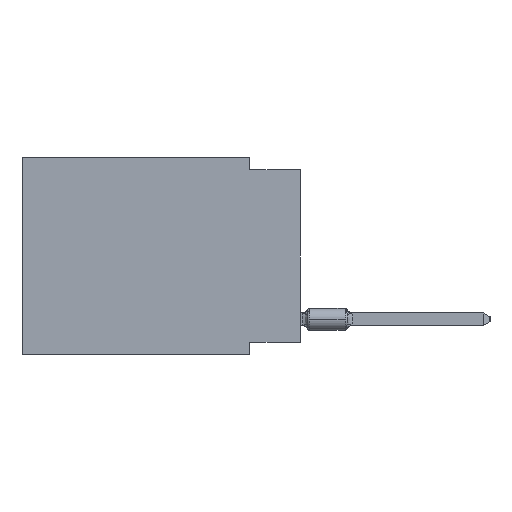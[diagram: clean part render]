
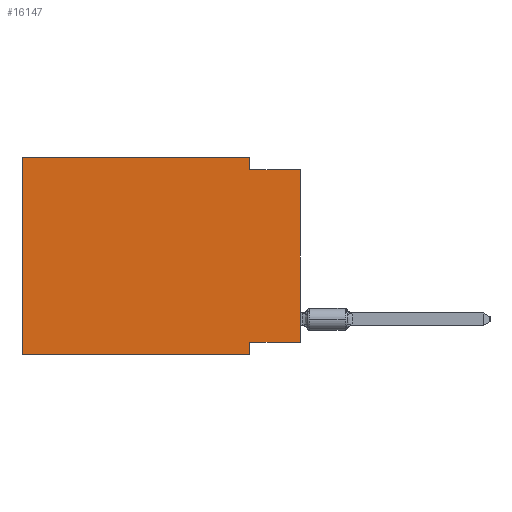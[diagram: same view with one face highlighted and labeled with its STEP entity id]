
A CAD part, left-side view. The second image highlights one B-rep face of the part: STEP entity #16147.
In plain terms, the highlighted planar face has unit normal (-1, 0, 0).
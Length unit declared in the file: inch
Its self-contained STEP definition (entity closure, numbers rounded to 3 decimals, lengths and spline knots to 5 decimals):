
#1 = VERTEX_POINT ( 'NONE', #627 ) ;
#300 = VECTOR ( 'NONE', #22819, 39.37008 ) ;
#627 = CARTESIAN_POINT ( 'NONE',  ( 0., 0., -0.365 ) ) ;
#1776 = VECTOR ( 'NONE', #17941, 39.37008 ) ;
#2031 = CARTESIAN_POINT ( 'NONE',  ( 0., 0., 0. ) ) ;
#2058 = EDGE_CURVE ( 'NONE', #35539, #40178, #32119, .T. ) ;
#3514 = CARTESIAN_POINT ( 'NONE',  ( 0., 0.55, -0.39 ) ) ;
#4453 = CARTESIAN_POINT ( 'NONE',  ( 0., 0., -0.025 ) ) ;
#4583 = VECTOR ( 'NONE', #8873, 39.37008 ) ;
#5083 = LINE ( 'NONE', #16322, #5410 ) ;
#5410 = VECTOR ( 'NONE', #23696, 39.37008 ) ;
#5437 = EDGE_LOOP ( 'NONE', ( #15225, #14082, #42609, #17119, #17878, #28107, #40906, #35796 ) ) ;
#6284 = VERTEX_POINT ( 'NONE', #42883 ) ;
#7705 = CARTESIAN_POINT ( 'NONE',  ( 0., 0., -0.365 ) ) ;
#7922 = LINE ( 'NONE', #38266, #4583 ) ;
#8873 = DIRECTION ( 'NONE',  ( 0., 0., 1. ) ) ;
#10117 = LINE ( 'NONE', #2031, #1776 ) ;
#10645 = DIRECTION ( 'NONE',  ( 1., 0., 0. ) ) ;
#10716 = VECTOR ( 'NONE', #33908, 39.37008 ) ;
#11028 = EDGE_CURVE ( 'NONE', #46949, #6284, #14076, .T. ) ;
#11134 = EDGE_CURVE ( 'NONE', #1, #34739, #41002, .T. ) ;
#11147 = DIRECTION ( 'NONE',  ( 0., 0., -1. ) ) ;
#11807 = LINE ( 'NONE', #4453, #29707 ) ;
#11814 = VERTEX_POINT ( 'NONE', #28180 ) ;
#13243 = AXIS2_PLACEMENT_3D ( 'NONE', #36600, #10645, #11147 ) ;
#13517 = CARTESIAN_POINT ( 'NONE',  ( 0., 0.55, 0. ) ) ;
#14076 = LINE ( 'NONE', #39128, #23219 ) ;
#14082 = ORIENTED_EDGE ( 'NONE', *, *, #37525, .F. ) ;
#14322 = FACE_OUTER_BOUND ( 'NONE', #5437, .T. ) ;
#15012 = CARTESIAN_POINT ( 'NONE',  ( 0., 0.1, -0.365 ) ) ;
#15225 = ORIENTED_EDGE ( 'NONE', *, *, #47843, .T. ) ;
#16147 = ADVANCED_FACE ( 'NONE', ( #14322 ), #21663, .F. ) ;
#16322 = CARTESIAN_POINT ( 'NONE',  ( 0., 0.1, -0.39 ) ) ;
#17119 = ORIENTED_EDGE ( 'NONE', *, *, #2058, .F. ) ;
#17878 = ORIENTED_EDGE ( 'NONE', *, *, #36021, .F. ) ;
#17884 = VECTOR ( 'NONE', #47873, 39.37008 ) ;
#17941 = DIRECTION ( 'NONE',  ( 0., 0., 1. ) ) ;
#19382 = DIRECTION ( 'NONE',  ( 0., -1., 0. ) ) ;
#20889 = CARTESIAN_POINT ( 'NONE',  ( 0., 0.1, 0. ) ) ;
#21663 = PLANE ( 'NONE',  #13243 ) ;
#22648 = LINE ( 'NONE', #41009, #17884 ) ;
#22819 = DIRECTION ( 'NONE',  ( 0., -1., 0. ) ) ;
#23219 = VECTOR ( 'NONE', #35225, 39.37008 ) ;
#23696 = DIRECTION ( 'NONE',  ( 0., 0., -1. ) ) ;
#24435 = VERTEX_POINT ( 'NONE', #47592 ) ;
#28107 = ORIENTED_EDGE ( 'NONE', *, *, #11028, .T. ) ;
#28180 = CARTESIAN_POINT ( 'NONE',  ( 0., 0.1, -0.025 ) ) ;
#29707 = VECTOR ( 'NONE', #19382, 39.37008 ) ;
#32119 = LINE ( 'NONE', #13517, #300 ) ;
#33908 = DIRECTION ( 'NONE',  ( 0., 1., 0. ) ) ;
#34339 = EDGE_CURVE ( 'NONE', #40178, #11814, #22648, .T. ) ;
#34739 = VERTEX_POINT ( 'NONE', #15012 ) ;
#35225 = DIRECTION ( 'NONE',  ( 0., -1., 0. ) ) ;
#35228 = EDGE_CURVE ( 'NONE', #34739, #6284, #5083, .T. ) ;
#35539 = VERTEX_POINT ( 'NONE', #37347 ) ;
#35796 = ORIENTED_EDGE ( 'NONE', *, *, #11134, .F. ) ;
#36021 = EDGE_CURVE ( 'NONE', #46949, #35539, #7922, .T. ) ;
#36600 = CARTESIAN_POINT ( 'NONE',  ( 0., 0.55, 0. ) ) ;
#37347 = CARTESIAN_POINT ( 'NONE',  ( 0., 0.55, 0. ) ) ;
#37525 = EDGE_CURVE ( 'NONE', #11814, #24435, #11807, .T. ) ;
#38266 = CARTESIAN_POINT ( 'NONE',  ( 0., 0.55, 0. ) ) ;
#39128 = CARTESIAN_POINT ( 'NONE',  ( 0., 0.55, -0.39 ) ) ;
#40178 = VERTEX_POINT ( 'NONE', #20889 ) ;
#40906 = ORIENTED_EDGE ( 'NONE', *, *, #35228, .F. ) ;
#41002 = LINE ( 'NONE', #7705, #10716 ) ;
#41009 = CARTESIAN_POINT ( 'NONE',  ( 0., 0.1, 0. ) ) ;
#42609 = ORIENTED_EDGE ( 'NONE', *, *, #34339, .F. ) ;
#42883 = CARTESIAN_POINT ( 'NONE',  ( 0., 0.1, -0.39 ) ) ;
#46949 = VERTEX_POINT ( 'NONE', #3514 ) ;
#47592 = CARTESIAN_POINT ( 'NONE',  ( 0., 0., -0.025 ) ) ;
#47843 = EDGE_CURVE ( 'NONE', #1, #24435, #10117, .T. ) ;
#47873 = DIRECTION ( 'NONE',  ( 0., 0., -1. ) ) ;
